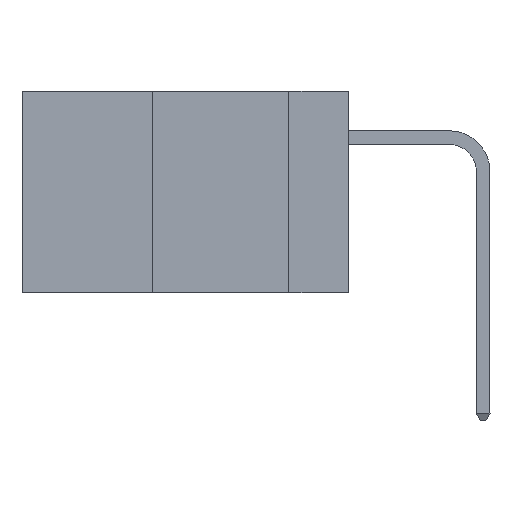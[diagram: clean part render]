
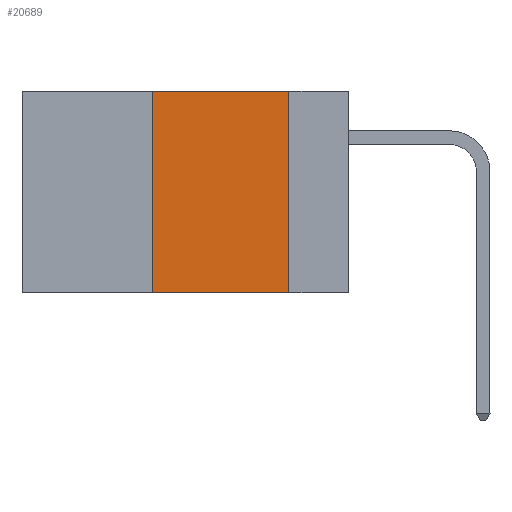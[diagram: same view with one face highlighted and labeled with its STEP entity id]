
A CAD part, left-side view. The second image highlights one B-rep face of the part: STEP entity #20689.
In plain terms, the highlighted planar face has unit normal (-1, 0, 0).
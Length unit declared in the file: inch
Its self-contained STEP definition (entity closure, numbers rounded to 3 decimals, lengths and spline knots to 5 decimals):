
#356 = DIRECTION ( 'NONE',  ( 0., 0., -1. ) ) ;
#726 = VERTEX_POINT ( 'NONE', #9701 ) ;
#802 = EDGE_CURVE ( 'NONE', #11286, #4987, #17480, .T. ) ;
#1000 = LINE ( 'NONE', #2271, #20321 ) ;
#1260 = CARTESIAN_POINT ( 'NONE',  ( 0., 0.11, -0.37 ) ) ;
#2271 = CARTESIAN_POINT ( 'NONE',  ( 0., 0.36, 0. ) ) ;
#2998 = ORIENTED_EDGE ( 'NONE', *, *, #6194, .F. ) ;
#3851 = PLANE ( 'NONE',  #12893 ) ;
#4987 = VERTEX_POINT ( 'NONE', #1260 ) ;
#5249 = DIRECTION ( 'NONE',  ( 1., 0., 0. ) ) ;
#5552 = EDGE_LOOP ( 'NONE', ( #16558, #18159, #2998, #14014 ) ) ;
#6194 = EDGE_CURVE ( 'NONE', #11286, #726, #1000, .T. ) ;
#7258 = CARTESIAN_POINT ( 'NONE',  ( 0., 0.11, 0. ) ) ;
#7721 = EDGE_CURVE ( 'NONE', #18890, #4987, #14111, .T. ) ;
#9701 = CARTESIAN_POINT ( 'NONE',  ( 0., 0.36, 0. ) ) ;
#10050 = CARTESIAN_POINT ( 'NONE',  ( 0., 0.11, 0. ) ) ;
#10184 = CARTESIAN_POINT ( 'NONE',  ( 0., 0.6, 0. ) ) ;
#10296 = DIRECTION ( 'NONE',  ( 0., -1., 0. ) ) ;
#11286 = VERTEX_POINT ( 'NONE', #17205 ) ;
#11883 = DIRECTION ( 'NONE',  ( 0., -1., 0. ) ) ;
#12893 = AXIS2_PLACEMENT_3D ( 'NONE', #14079, #5249, #356 ) ;
#14014 = ORIENTED_EDGE ( 'NONE', *, *, #802, .T. ) ;
#14079 = CARTESIAN_POINT ( 'NONE',  ( 0., 0.6, 0. ) ) ;
#14111 = LINE ( 'NONE', #7258, #21862 ) ;
#15941 = FACE_OUTER_BOUND ( 'NONE', #5552, .T. ) ;
#16558 = ORIENTED_EDGE ( 'NONE', *, *, #7721, .F. ) ;
#16692 = DIRECTION ( 'NONE',  ( 0., 0., 1. ) ) ;
#16784 = VECTOR ( 'NONE', #11883, 39.37008 ) ;
#17137 = CARTESIAN_POINT ( 'NONE',  ( 0., 0.6, -0.37 ) ) ;
#17182 = EDGE_CURVE ( 'NONE', #726, #18890, #20350, .T. ) ;
#17205 = CARTESIAN_POINT ( 'NONE',  ( 0., 0.36, -0.37 ) ) ;
#17480 = LINE ( 'NONE', #17137, #16784 ) ;
#17982 = VECTOR ( 'NONE', #10296, 39.37008 ) ;
#18159 = ORIENTED_EDGE ( 'NONE', *, *, #17182, .F. ) ;
#18890 = VERTEX_POINT ( 'NONE', #10050 ) ;
#20321 = VECTOR ( 'NONE', #16692, 39.37008 ) ;
#20350 = LINE ( 'NONE', #10184, #17982 ) ;
#20689 = ADVANCED_FACE ( 'NONE', ( #15941 ), #3851, .F. ) ;
#21552 = DIRECTION ( 'NONE',  ( 0., 0., -1. ) ) ;
#21862 = VECTOR ( 'NONE', #21552, 39.37008 ) ;
